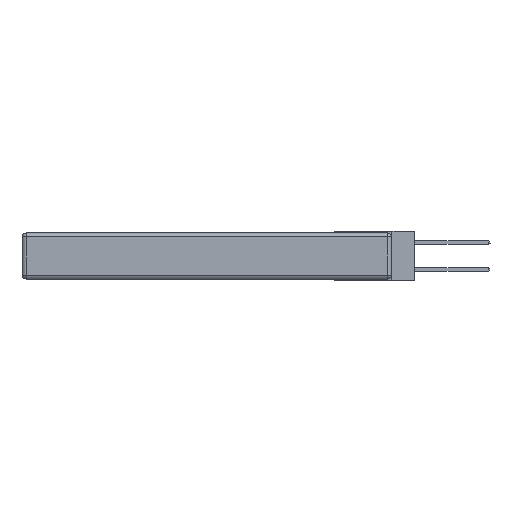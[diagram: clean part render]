
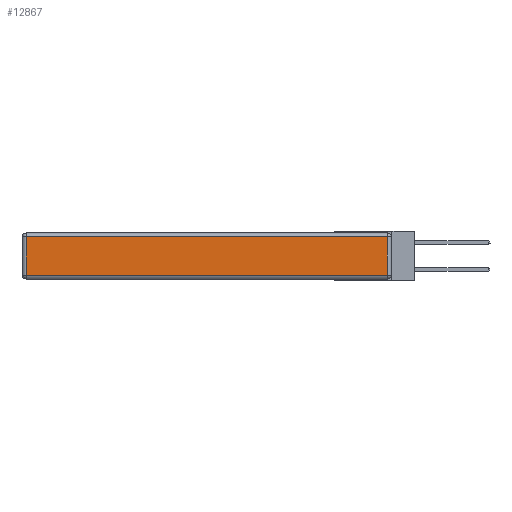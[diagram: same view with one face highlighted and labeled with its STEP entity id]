
A CAD part, left-side view. The second image highlights one B-rep face of the part: STEP entity #12867.
In plain terms, the highlighted planar face has unit normal (-1, 0, 0).
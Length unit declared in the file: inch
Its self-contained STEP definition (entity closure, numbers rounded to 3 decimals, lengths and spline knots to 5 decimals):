
#589 = VERTEX_POINT ( 'NONE', #7294 ) ;
#603 = PLANE ( 'NONE',  #3447 ) ;
#898 = VECTOR ( 'NONE', #14089, 39.37008 ) ;
#1831 = CARTESIAN_POINT ( 'NONE',  ( 0., 0., -0.313 ) ) ;
#2736 = EDGE_CURVE ( 'NONE', #11624, #19201, #20151, .T. ) ;
#3326 = EDGE_CURVE ( 'NONE', #8336, #589, #17568, .T. ) ;
#3447 = AXIS2_PLACEMENT_3D ( 'NONE', #13663, #10338, #12066 ) ;
#3485 = CARTESIAN_POINT ( 'NONE',  ( 0., 2.75, -0.03 ) ) ;
#6994 = LINE ( 'NONE', #3485, #14167 ) ;
#7072 = FACE_OUTER_BOUND ( 'NONE', #16576, .T. ) ;
#7294 = CARTESIAN_POINT ( 'NONE',  ( 0., 0.03, -0.03 ) ) ;
#8295 = VECTOR ( 'NONE', #20630, 39.37008 ) ;
#8336 = VERTEX_POINT ( 'NONE', #21179 ) ;
#10338 = DIRECTION ( 'NONE',  ( -1., 0., 0. ) ) ;
#11624 = VERTEX_POINT ( 'NONE', #13273 ) ;
#11706 = DIRECTION ( 'NONE',  ( 0., -1., 0. ) ) ;
#12066 = DIRECTION ( 'NONE',  ( 0., 0., 1. ) ) ;
#12314 = ORIENTED_EDGE ( 'NONE', *, *, #3326, .T. ) ;
#12342 = CARTESIAN_POINT ( 'NONE',  ( 0., 0.03, -0.343 ) ) ;
#12591 = ORIENTED_EDGE ( 'NONE', *, *, #14504, .T. ) ;
#12867 = ADVANCED_FACE ( 'NONE', ( #7072 ), #603, .T. ) ;
#13273 = CARTESIAN_POINT ( 'NONE',  ( 0., 2.72, -0.03 ) ) ;
#13663 = CARTESIAN_POINT ( 'NONE',  ( 0., 0., -0.343 ) ) ;
#13810 = DIRECTION ( 'NONE',  ( 0., 1., 0. ) ) ;
#13943 = ORIENTED_EDGE ( 'NONE', *, *, #2736, .T. ) ;
#14089 = DIRECTION ( 'NONE',  ( 0., 0., -1. ) ) ;
#14167 = VECTOR ( 'NONE', #13810, 39.37008 ) ;
#14224 = CARTESIAN_POINT ( 'NONE',  ( 0., 2.72, -0.343 ) ) ;
#14383 = EDGE_CURVE ( 'NONE', #19201, #8336, #19835, .T. ) ;
#14504 = EDGE_CURVE ( 'NONE', #589, #11624, #6994, .T. ) ;
#16576 = EDGE_LOOP ( 'NONE', ( #17663, #12314, #12591, #13943 ) ) ;
#17568 = LINE ( 'NONE', #12342, #8295 ) ;
#17663 = ORIENTED_EDGE ( 'NONE', *, *, #14383, .T. ) ;
#19201 = VERTEX_POINT ( 'NONE', #19290 ) ;
#19290 = CARTESIAN_POINT ( 'NONE',  ( 0., 2.72, -0.313 ) ) ;
#19591 = VECTOR ( 'NONE', #11706, 39.37008 ) ;
#19835 = LINE ( 'NONE', #1831, #19591 ) ;
#20151 = LINE ( 'NONE', #14224, #898 ) ;
#20630 = DIRECTION ( 'NONE',  ( 0., 0., 1. ) ) ;
#21179 = CARTESIAN_POINT ( 'NONE',  ( 0., 0.03, -0.313 ) ) ;
